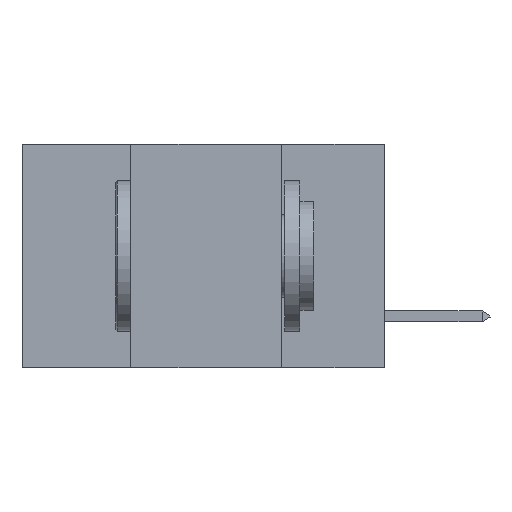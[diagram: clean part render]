
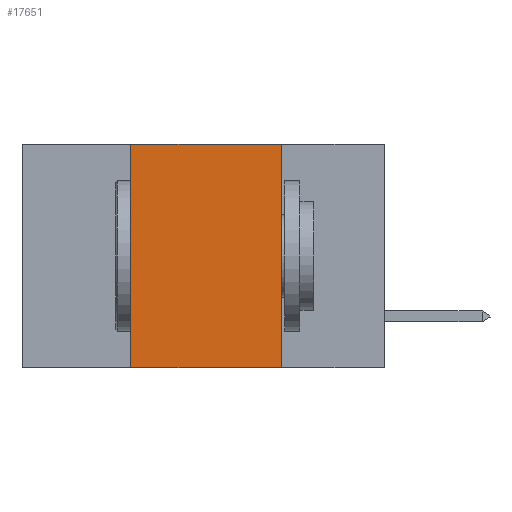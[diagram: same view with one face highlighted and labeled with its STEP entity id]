
A CAD part, left-side view. The second image highlights one B-rep face of the part: STEP entity #17651.
In plain terms, the highlighted planar face has unit normal (-1, 0, 0).
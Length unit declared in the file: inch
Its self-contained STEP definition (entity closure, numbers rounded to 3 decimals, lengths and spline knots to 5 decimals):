
#456 = EDGE_CURVE ( 'NONE', #36304, #26261, #3135, .T. ) ;
#1374 = VECTOR ( 'NONE', #13146, 39.37008 ) ;
#1937 = DIRECTION ( 'NONE',  ( 1., 0., 0. ) ) ;
#2785 = DIRECTION ( 'NONE',  ( 0., 0., -1. ) ) ;
#3135 = LINE ( 'NONE', #34563, #29211 ) ;
#3989 = ORIENTED_EDGE ( 'NONE', *, *, #32259, .T. ) ;
#6511 = VECTOR ( 'NONE', #21199, 39.37008 ) ;
#7330 = CARTESIAN_POINT ( 'NONE',  ( 0., 0.17, -0.37 ) ) ;
#7787 = EDGE_CURVE ( 'NONE', #36053, #20133, #30738, .T. ) ;
#8863 = CARTESIAN_POINT ( 'NONE',  ( 0., 0.17, 0. ) ) ;
#9888 = LINE ( 'NONE', #24953, #1374 ) ;
#10399 = FACE_OUTER_BOUND ( 'NONE', #38514, .T. ) ;
#11820 = CARTESIAN_POINT ( 'NONE',  ( 0., 0.6, 0. ) ) ;
#11961 = ORIENTED_EDGE ( 'NONE', *, *, #32779, .F. ) ;
#13146 = DIRECTION ( 'NONE',  ( 0., -1., 0. ) ) ;
#16382 = DIRECTION ( 'NONE',  ( 0., 0., 1. ) ) ;
#17651 = ADVANCED_FACE ( 'NONE', ( #10399 ), #26178, .F. ) ;
#20133 = VERTEX_POINT ( 'NONE', #7330 ) ;
#21199 = DIRECTION ( 'NONE',  ( 0., -1., 0. ) ) ;
#23273 = CARTESIAN_POINT ( 'NONE',  ( 0., 0.6, 0. ) ) ;
#24953 = CARTESIAN_POINT ( 'NONE',  ( 0., 0.6, -0.37 ) ) ;
#26178 = PLANE ( 'NONE',  #36831 ) ;
#26261 = VERTEX_POINT ( 'NONE', #34251 ) ;
#26869 = ORIENTED_EDGE ( 'NONE', *, *, #456, .F. ) ;
#28318 = CARTESIAN_POINT ( 'NONE',  ( 0., 0.17, 0. ) ) ;
#29211 = VECTOR ( 'NONE', #16382, 39.37008 ) ;
#29485 = DIRECTION ( 'NONE',  ( 0., 0., -1. ) ) ;
#29507 = CARTESIAN_POINT ( 'NONE',  ( 0., 0.42, -0.37 ) ) ;
#30252 = VECTOR ( 'NONE', #2785, 39.37008 ) ;
#30738 = LINE ( 'NONE', #8863, #30252 ) ;
#31173 = LINE ( 'NONE', #11820, #6511 ) ;
#32259 = EDGE_CURVE ( 'NONE', #36304, #20133, #9888, .T. ) ;
#32779 = EDGE_CURVE ( 'NONE', #26261, #36053, #31173, .T. ) ;
#34251 = CARTESIAN_POINT ( 'NONE',  ( 0., 0.42, 0. ) ) ;
#34563 = CARTESIAN_POINT ( 'NONE',  ( 0., 0.42, 0. ) ) ;
#35718 = ORIENTED_EDGE ( 'NONE', *, *, #7787, .F. ) ;
#36053 = VERTEX_POINT ( 'NONE', #28318 ) ;
#36304 = VERTEX_POINT ( 'NONE', #29507 ) ;
#36831 = AXIS2_PLACEMENT_3D ( 'NONE', #23273, #1937, #29485 ) ;
#38514 = EDGE_LOOP ( 'NONE', ( #35718, #11961, #26869, #3989 ) ) ;
